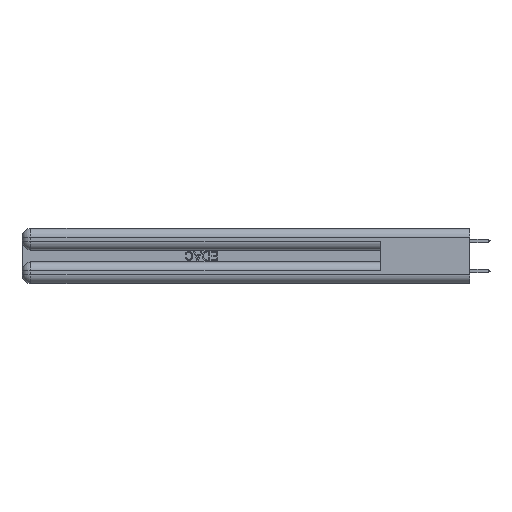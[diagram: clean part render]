
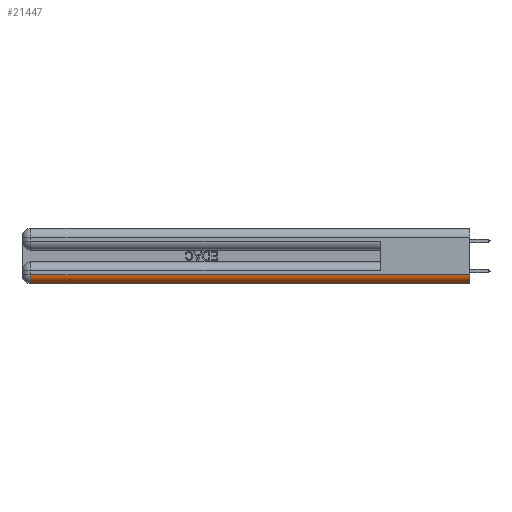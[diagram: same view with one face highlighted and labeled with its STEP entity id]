
A CAD part, left-side view. The second image highlights one B-rep face of the part: STEP entity #21447.
In plain terms, the highlighted cylindrical face has radius 1.524 mm (diameter 3.048 mm), a partial arc.
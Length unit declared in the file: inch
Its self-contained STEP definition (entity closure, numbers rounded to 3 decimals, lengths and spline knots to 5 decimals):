
#1048 = FACE_OUTER_BOUND ( 'NONE', #3706, .T. ) ;
#1410 = CARTESIAN_POINT ( 'NONE',  ( 0., 0., 0.06 ) ) ;
#2182 = CARTESIAN_POINT ( 'NONE',  ( 0.06, 0., 0. ) ) ;
#3706 = EDGE_LOOP ( 'NONE', ( #39986, #16137, #18990, #11703 ) ) ;
#5038 = VERTEX_POINT ( 'NONE', #1410 ) ;
#5553 = VERTEX_POINT ( 'NONE', #14298 ) ;
#5796 = DIRECTION ( 'NONE',  ( 0., 1., 0. ) ) ;
#7410 = EDGE_CURVE ( 'NONE', #20822, #5553, #30424, .T. ) ;
#9275 = DIRECTION ( 'NONE',  ( 0., 1., 0. ) ) ;
#11357 = CARTESIAN_POINT ( 'NONE',  ( 0.06, 0., 0.06 ) ) ;
#11703 = ORIENTED_EDGE ( 'NONE', *, *, #7410, .F. ) ;
#12175 = CARTESIAN_POINT ( 'NONE',  ( 0.06, 3., 0. ) ) ;
#12608 = CARTESIAN_POINT ( 'NONE',  ( 0., 2.94, 0.06 ) ) ;
#12761 = AXIS2_PLACEMENT_3D ( 'NONE', #23575, #5796, #41072 ) ;
#14298 = CARTESIAN_POINT ( 'NONE',  ( 0.06, 2.94, 0. ) ) ;
#16137 = ORIENTED_EDGE ( 'NONE', *, *, #30332, .F. ) ;
#18990 = ORIENTED_EDGE ( 'NONE', *, *, #29758, .F. ) ;
#20822 = VERTEX_POINT ( 'NONE', #2182 ) ;
#20911 = VECTOR ( 'NONE', #39179, 39.37008 ) ;
#21447 = ADVANCED_FACE ( 'NONE', ( #1048 ), #35606, .T. ) ;
#23575 = CARTESIAN_POINT ( 'NONE',  ( 0.06, 0., 0.06 ) ) ;
#23660 = CARTESIAN_POINT ( 'NONE',  ( 0., 0., 0.06 ) ) ;
#24812 = DIRECTION ( 'NONE',  ( 0., 0., 1. ) ) ;
#26375 = AXIS2_PLACEMENT_3D ( 'NONE', #41071, #9275, #24812 ) ;
#27465 = DIRECTION ( 'NONE',  ( 0., -1., 0. ) ) ;
#27594 = DIRECTION ( 'NONE',  ( 0., 0., 1. ) ) ;
#29758 = EDGE_CURVE ( 'NONE', #5553, #33024, #37817, .T. ) ;
#30332 = EDGE_CURVE ( 'NONE', #33024, #5038, #35758, .T. ) ;
#30424 = LINE ( 'NONE', #12175, #20911 ) ;
#32282 = VECTOR ( 'NONE', #36562, 39.37008 ) ;
#33024 = VERTEX_POINT ( 'NONE', #12608 ) ;
#34475 = CIRCLE ( 'NONE', #38329, 0.06 ) ;
#34655 = EDGE_CURVE ( 'NONE', #5038, #20822, #34475, .T. ) ;
#35606 = CYLINDRICAL_SURFACE ( 'NONE', #12761, 0.06 ) ;
#35758 = LINE ( 'NONE', #23660, #32282 ) ;
#36562 = DIRECTION ( 'NONE',  ( 0., -1., 0. ) ) ;
#37817 = CIRCLE ( 'NONE', #26375, 0.06 ) ;
#38329 = AXIS2_PLACEMENT_3D ( 'NONE', #11357, #27465, #27594 ) ;
#39179 = DIRECTION ( 'NONE',  ( 0., 1., 0. ) ) ;
#39986 = ORIENTED_EDGE ( 'NONE', *, *, #34655, .F. ) ;
#41071 = CARTESIAN_POINT ( 'NONE',  ( 0.06, 2.94, 0.06 ) ) ;
#41072 = DIRECTION ( 'NONE',  ( 0., 0., 1. ) ) ;
